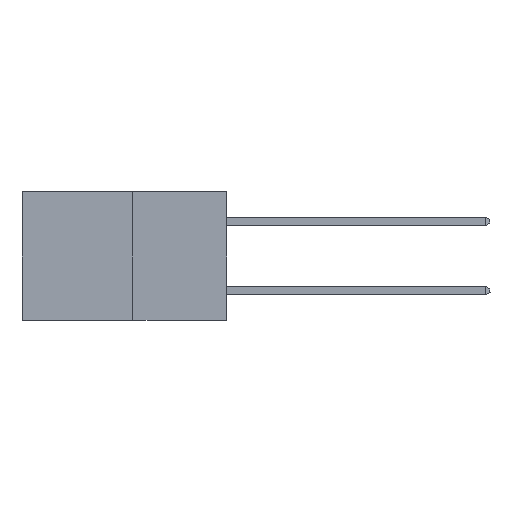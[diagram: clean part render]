
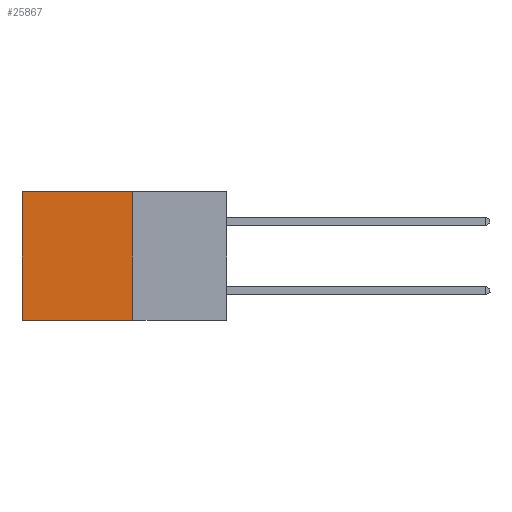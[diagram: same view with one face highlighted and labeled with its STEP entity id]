
A CAD part, left-side view. The second image highlights one B-rep face of the part: STEP entity #25867.
In plain terms, the highlighted planar face has unit normal (-1, 0, 0).
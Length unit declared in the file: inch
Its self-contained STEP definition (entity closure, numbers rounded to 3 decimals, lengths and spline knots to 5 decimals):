
#45 = ORIENTED_EDGE ( 'NONE', *, *, #14284, .F. ) ;
#975 = CARTESIAN_POINT ( 'NONE',  ( 0.277, 0.59, 0. ) ) ;
#2395 = LINE ( 'NONE', #23441, #14668 ) ;
#3843 = EDGE_CURVE ( 'NONE', #20788, #18379, #16822, .T. ) ;
#4529 = LINE ( 'NONE', #20962, #23186 ) ;
#6497 = PLANE ( 'NONE',  #29812 ) ;
#7226 = DIRECTION ( 'NONE',  ( 0., 1., 0. ) ) ;
#8281 = VERTEX_POINT ( 'NONE', #18489 ) ;
#8959 = CARTESIAN_POINT ( 'NONE',  ( 0.277, 0.27, -0.37 ) ) ;
#10220 = LINE ( 'NONE', #23709, #28804 ) ;
#10825 = EDGE_CURVE ( 'NONE', #18379, #8281, #2395, .T. ) ;
#11637 = DIRECTION ( 'NONE',  ( 0., 0., -1. ) ) ;
#14284 = EDGE_CURVE ( 'NONE', #20788, #28770, #10220, .T. ) ;
#14668 = VECTOR ( 'NONE', #25901, 39.37008 ) ;
#14772 = ORIENTED_EDGE ( 'NONE', *, *, #3843, .T. ) ;
#16297 = DIRECTION ( 'NONE',  ( 0., 0., -1. ) ) ;
#16822 = LINE ( 'NONE', #17728, #21731 ) ;
#17728 = CARTESIAN_POINT ( 'NONE',  ( 0.277, 0.27, 0. ) ) ;
#18379 = VERTEX_POINT ( 'NONE', #975 ) ;
#18489 = CARTESIAN_POINT ( 'NONE',  ( 0.277, 0.59, -0.37 ) ) ;
#20788 = VERTEX_POINT ( 'NONE', #30380 ) ;
#20962 = CARTESIAN_POINT ( 'NONE',  ( 0.277, 0.27, -0.37 ) ) ;
#21665 = FACE_OUTER_BOUND ( 'NONE', #22880, .T. ) ;
#21731 = VECTOR ( 'NONE', #7226, 39.37008 ) ;
#22507 = ORIENTED_EDGE ( 'NONE', *, *, #10825, .T. ) ;
#22880 = EDGE_LOOP ( 'NONE', ( #22507, #27957, #45, #14772 ) ) ;
#23186 = VECTOR ( 'NONE', #28261, 39.37008 ) ;
#23441 = CARTESIAN_POINT ( 'NONE',  ( 0.277, 0.59, -0.37 ) ) ;
#23709 = CARTESIAN_POINT ( 'NONE',  ( 0.277, 0.27, -0.37 ) ) ;
#25825 = EDGE_CURVE ( 'NONE', #28770, #8281, #4529, .T. ) ;
#25867 = ADVANCED_FACE ( 'NONE', ( #21665 ), #6497, .F. ) ;
#25901 = DIRECTION ( 'NONE',  ( 0., 0., -1. ) ) ;
#27957 = ORIENTED_EDGE ( 'NONE', *, *, #25825, .F. ) ;
#28040 = CARTESIAN_POINT ( 'NONE',  ( 0.277, 0.27, -0.37 ) ) ;
#28261 = DIRECTION ( 'NONE',  ( 0., 1., 0. ) ) ;
#28770 = VERTEX_POINT ( 'NONE', #28040 ) ;
#28804 = VECTOR ( 'NONE', #11637, 39.37008 ) ;
#29812 = AXIS2_PLACEMENT_3D ( 'NONE', #8959, #30821, #16297 ) ;
#30380 = CARTESIAN_POINT ( 'NONE',  ( 0.277, 0.27, 0. ) ) ;
#30821 = DIRECTION ( 'NONE',  ( 1., 0., 0. ) ) ;
